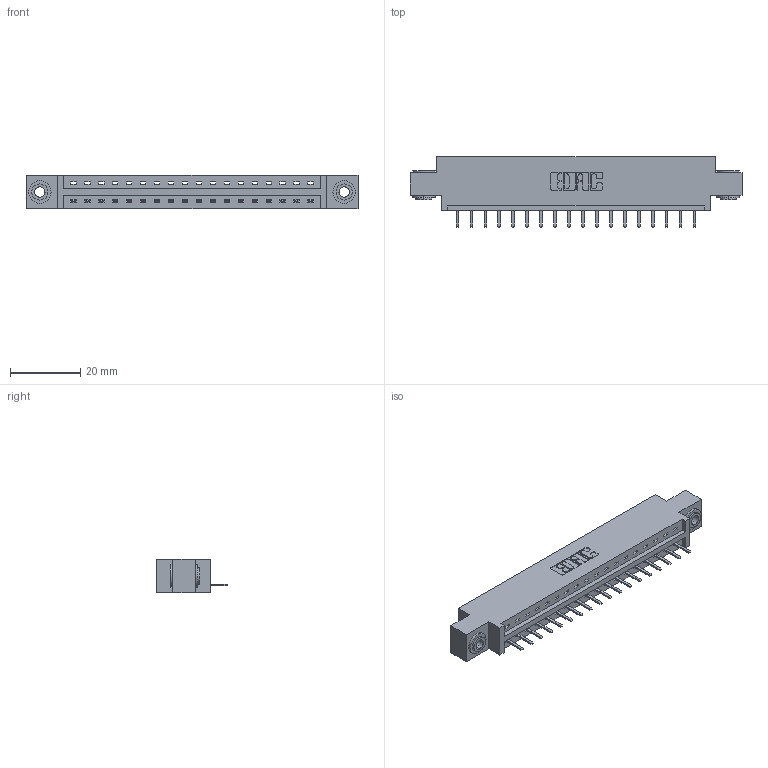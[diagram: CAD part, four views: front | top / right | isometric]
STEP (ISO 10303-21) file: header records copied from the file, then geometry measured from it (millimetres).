
FILE_DESCRIPTION (( 'STEP AP203' ), '1' );
FILE_NAME ('337-018-520-603.STEP', '2019-09-28T19:38:10', ( '' ), ( '' ), 'SwSTEP 2.0', 'SolidWorks 2016', '' );
FILE_SCHEMA (( 'CONFIG_CONTROL_DESIGN' ));
Length unit declared in the file: inch
Products named in the file (4): 337-018-520-603; 345-292-001_345-293-120; 345-250-002_345-250-002-102; 337 Part_0.170 Offset - 0.156 Dia-TH
Assembly tree (21 placements, depth 2):
  337-018-520-603
    337 Part_0.170 Offset - 0.156 Dia-TH
    345-292-001_345-293-120  x18
    345-250-002_345-250-002-102  x2
Bounding box: 94.34 x 20.02 x 9.4 mm (x, y, z)
Volume: 9354.4 mm3; surface area: 9675.9 mm2
Topology: 21 solids, 21 shells, 1344 faces, 3927 edges, 2566 vertices
Faces by surface type: plane 948, cylinder 388, cone 8
Entity records: 17380 total; most frequent: CARTESIAN_POINT 3015, ORIENTED_EDGE 2950, DIRECTION 2609, EDGE_CURVE 1475, LINE 1319, VECTOR 1319, VERTEX_POINT 978, AXIS2_PLACEMENT_3D 645
